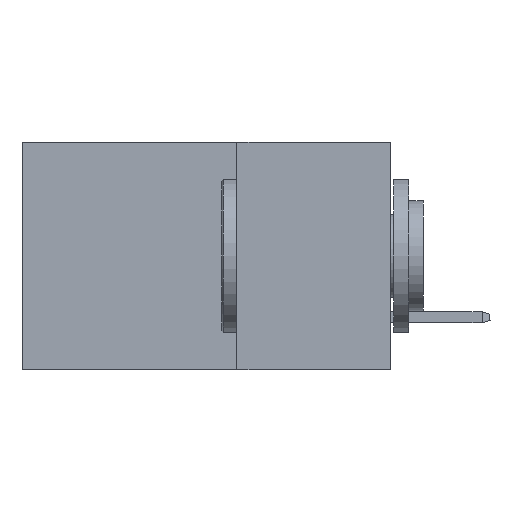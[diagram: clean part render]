
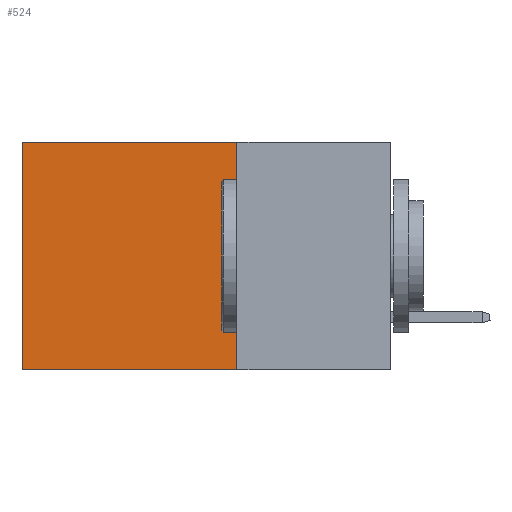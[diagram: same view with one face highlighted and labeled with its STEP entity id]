
A CAD part, left-side view. The second image highlights one B-rep face of the part: STEP entity #524.
In plain terms, the highlighted planar face has unit normal (-1, 0, 0).
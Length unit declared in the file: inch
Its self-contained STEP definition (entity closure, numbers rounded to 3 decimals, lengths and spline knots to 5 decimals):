
#524 = ADVANCED_FACE ( 'NONE', ( #14273 ), #15647, .F. ) ;
#1819 = LINE ( 'NONE', #16339, #11998 ) ;
#2281 = VECTOR ( 'NONE', #4626, 39.37008 ) ;
#4239 = DIRECTION ( 'NONE',  ( 0., 0., -1. ) ) ;
#4626 = DIRECTION ( 'NONE',  ( 0., 1., 0. ) ) ;
#6112 = CARTESIAN_POINT ( 'NONE',  ( 0.2875, 0.25, -0.37 ) ) ;
#6575 = EDGE_LOOP ( 'NONE', ( #14681, #8342, #7396, #15930 ) ) ;
#6698 = VERTEX_POINT ( 'NONE', #10800 ) ;
#7396 = ORIENTED_EDGE ( 'NONE', *, *, #9277, .F. ) ;
#8342 = ORIENTED_EDGE ( 'NONE', *, *, #8394, .F. ) ;
#8394 = EDGE_CURVE ( 'NONE', #10245, #6698, #16273, .T. ) ;
#9277 = EDGE_CURVE ( 'NONE', #18520, #10245, #12672, .T. ) ;
#10139 = VECTOR ( 'NONE', #13948, 39.37008 ) ;
#10245 = VERTEX_POINT ( 'NONE', #11941 ) ;
#10800 = CARTESIAN_POINT ( 'NONE',  ( 0.2875, 0.6, -0.37 ) ) ;
#10833 = CARTESIAN_POINT ( 'NONE',  ( 0.2875, 0.6, 0. ) ) ;
#10974 = CARTESIAN_POINT ( 'NONE',  ( 0.2875, 0.25, 0. ) ) ;
#11104 = LINE ( 'NONE', #10974, #10139 ) ;
#11941 = CARTESIAN_POINT ( 'NONE',  ( 0.2875, 0.25, -0.37 ) ) ;
#11998 = VECTOR ( 'NONE', #13332, 39.37008 ) ;
#12241 = CARTESIAN_POINT ( 'NONE',  ( 0.2875, 0.25, 0. ) ) ;
#12488 = DIRECTION ( 'NONE',  ( 0., 0., -1. ) ) ;
#12672 = LINE ( 'NONE', #18231, #14332 ) ;
#13332 = DIRECTION ( 'NONE',  ( 0., 0., -1. ) ) ;
#13948 = DIRECTION ( 'NONE',  ( 0., 1., 0. ) ) ;
#14273 = FACE_OUTER_BOUND ( 'NONE', #6575, .T. ) ;
#14332 = VECTOR ( 'NONE', #4239, 39.37008 ) ;
#14681 = ORIENTED_EDGE ( 'NONE', *, *, #17104, .T. ) ;
#15509 = DIRECTION ( 'NONE',  ( 1., 0., 0. ) ) ;
#15545 = VERTEX_POINT ( 'NONE', #10833 ) ;
#15561 = AXIS2_PLACEMENT_3D ( 'NONE', #19982, #15509, #12488 ) ;
#15647 = PLANE ( 'NONE',  #15561 ) ;
#15930 = ORIENTED_EDGE ( 'NONE', *, *, #17412, .T. ) ;
#16273 = LINE ( 'NONE', #6112, #2281 ) ;
#16339 = CARTESIAN_POINT ( 'NONE',  ( 0.2875, 0.6, 0. ) ) ;
#17104 = EDGE_CURVE ( 'NONE', #15545, #6698, #1819, .T. ) ;
#17412 = EDGE_CURVE ( 'NONE', #18520, #15545, #11104, .T. ) ;
#18231 = CARTESIAN_POINT ( 'NONE',  ( 0.2875, 0.25, 0. ) ) ;
#18520 = VERTEX_POINT ( 'NONE', #12241 ) ;
#19982 = CARTESIAN_POINT ( 'NONE',  ( 0.2875, 0.25, 0. ) ) ;
